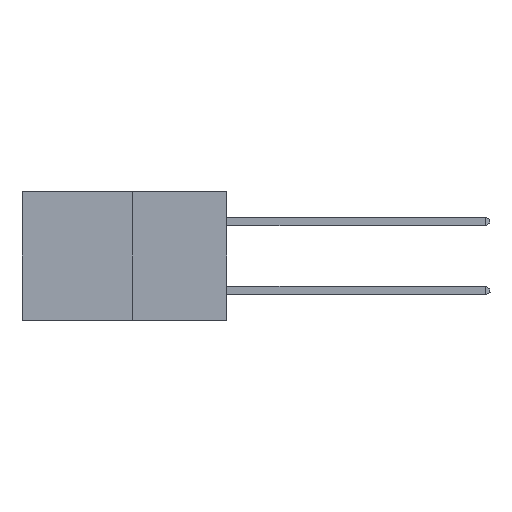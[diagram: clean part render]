
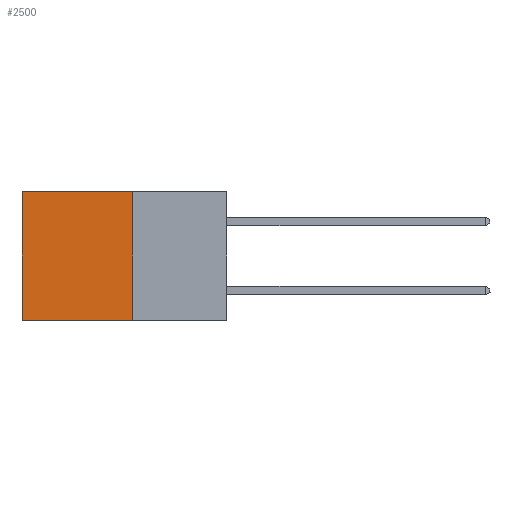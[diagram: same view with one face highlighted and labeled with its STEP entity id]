
A CAD part, left-side view. The second image highlights one B-rep face of the part: STEP entity #2500.
In plain terms, the highlighted planar face has unit normal (-1, 0, 0).
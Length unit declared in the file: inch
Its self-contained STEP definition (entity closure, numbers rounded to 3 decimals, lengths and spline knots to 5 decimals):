
#260 = VERTEX_POINT ( 'NONE', #9574 ) ;
#487 = LINE ( 'NONE', #7443, #9074 ) ;
#599 = ORIENTED_EDGE ( 'NONE', *, *, #8008, .T. ) ;
#993 = VECTOR ( 'NONE', #2308, 39.37008 ) ;
#1005 = CARTESIAN_POINT ( 'NONE',  ( 0.277, 0.27, 0. ) ) ;
#1084 = LINE ( 'NONE', #1005, #7391 ) ;
#1533 = LINE ( 'NONE', #7033, #993 ) ;
#1785 = CARTESIAN_POINT ( 'NONE',  ( 0.277, 0.27, 0. ) ) ;
#2296 = ORIENTED_EDGE ( 'NONE', *, *, #3257, .F. ) ;
#2308 = DIRECTION ( 'NONE',  ( 0., 0., -1. ) ) ;
#2500 = ADVANCED_FACE ( 'NONE', ( #9955 ), #4898, .F. ) ;
#2872 = VECTOR ( 'NONE', #7233, 39.37008 ) ;
#3023 = VERTEX_POINT ( 'NONE', #3189 ) ;
#3189 = CARTESIAN_POINT ( 'NONE',  ( 0.277, 0.27, -0.37 ) ) ;
#3257 = EDGE_CURVE ( 'NONE', #6071, #3023, #5068, .T. ) ;
#3346 = AXIS2_PLACEMENT_3D ( 'NONE', #6943, #4254, #3441 ) ;
#3441 = DIRECTION ( 'NONE',  ( 0., 0., -1. ) ) ;
#4094 = VERTEX_POINT ( 'NONE', #10007 ) ;
#4254 = DIRECTION ( 'NONE',  ( 1., 0., 0. ) ) ;
#4769 = EDGE_CURVE ( 'NONE', #260, #4094, #1533, .T. ) ;
#4898 = PLANE ( 'NONE',  #3346 ) ;
#5068 = LINE ( 'NONE', #9576, #2872 ) ;
#6071 = VERTEX_POINT ( 'NONE', #1785 ) ;
#6809 = DIRECTION ( 'NONE',  ( 0., 1., 0. ) ) ;
#6829 = EDGE_LOOP ( 'NONE', ( #9586, #8371, #2296, #599 ) ) ;
#6943 = CARTESIAN_POINT ( 'NONE',  ( 0.277, 0.27, -0.37 ) ) ;
#7033 = CARTESIAN_POINT ( 'NONE',  ( 0.277, 0.59, -0.37 ) ) ;
#7233 = DIRECTION ( 'NONE',  ( 0., 0., -1. ) ) ;
#7391 = VECTOR ( 'NONE', #6809, 39.37008 ) ;
#7443 = CARTESIAN_POINT ( 'NONE',  ( 0.277, 0.27, -0.37 ) ) ;
#8008 = EDGE_CURVE ( 'NONE', #6071, #260, #1084, .T. ) ;
#8275 = DIRECTION ( 'NONE',  ( 0., 1., 0. ) ) ;
#8371 = ORIENTED_EDGE ( 'NONE', *, *, #9121, .F. ) ;
#9074 = VECTOR ( 'NONE', #8275, 39.37008 ) ;
#9121 = EDGE_CURVE ( 'NONE', #3023, #4094, #487, .T. ) ;
#9574 = CARTESIAN_POINT ( 'NONE',  ( 0.277, 0.59, 0. ) ) ;
#9576 = CARTESIAN_POINT ( 'NONE',  ( 0.277, 0.27, -0.37 ) ) ;
#9586 = ORIENTED_EDGE ( 'NONE', *, *, #4769, .T. ) ;
#9955 = FACE_OUTER_BOUND ( 'NONE', #6829, .T. ) ;
#10007 = CARTESIAN_POINT ( 'NONE',  ( 0.277, 0.59, -0.37 ) ) ;
